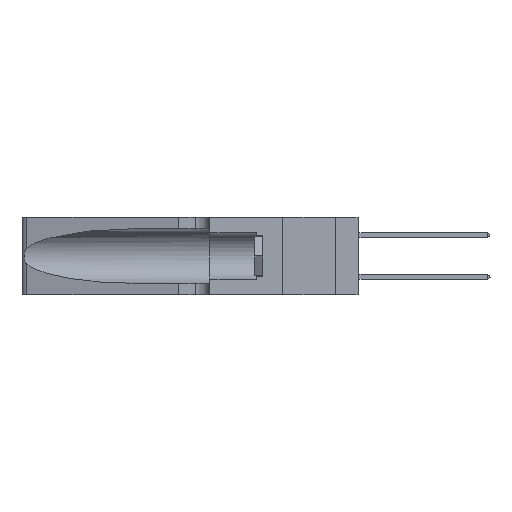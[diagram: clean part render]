
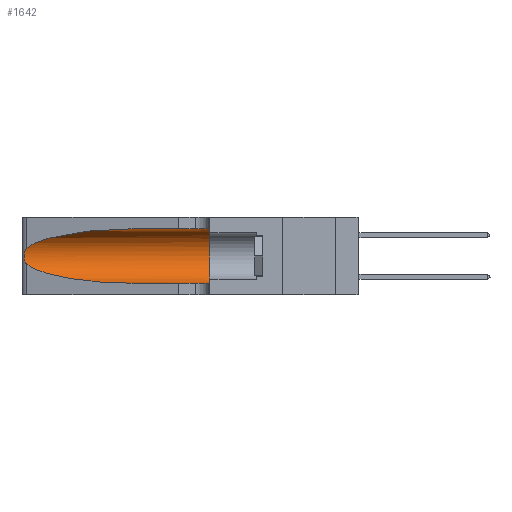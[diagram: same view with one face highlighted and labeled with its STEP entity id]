
A CAD part, left-side view. The second image highlights one B-rep face of the part: STEP entity #1642.
In plain terms, the highlighted cylindrical face has radius 3.308 mm (diameter 6.617 mm), a partial arc.
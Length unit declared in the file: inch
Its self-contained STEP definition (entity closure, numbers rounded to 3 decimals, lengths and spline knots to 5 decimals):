
#1467 = CARTESIAN_POINT ( 'NONE',  ( 0.25487, 1.22718, 0.14631 ) ) ;
#1642 = ADVANCED_FACE ( 'NONE', ( #1729 ), #6594, .F. ) ;
#1729 = FACE_OUTER_BOUND ( 'NONE', #39317, .T. ) ;
#2793 = CARTESIAN_POINT ( 'NONE',  ( 0.25856, 1.23593, 0.16098 ) ) ;
#3028 = EDGE_CURVE ( 'NONE', #35115, #24705, #32101, .T. ) ;
#3252 = CARTESIAN_POINT ( 'NONE',  ( 0.1305, 1.61858, 0.185 ) ) ;
#4493 = CARTESIAN_POINT ( 'NONE',  ( 0.25555, 1.22993, 0.14849 ) ) ;
#4665 = EDGE_CURVE ( 'NONE', #39613, #35115, #19788, .T. ) ;
#5432 = LINE ( 'NONE', #15049, #13195 ) ;
#6594 = CYLINDRICAL_SURFACE ( 'NONE', #13612, 0.13025 ) ;
#7009 =( BOUNDED_CURVE ( )  B_SPLINE_CURVE ( 3, ( #38324, #22607, #38751, #10418 ),
 .UNSPECIFIED., .F., .T. ) 
 B_SPLINE_CURVE_WITH_KNOTS ( ( 4, 4 ),
 ( 1.5708, 2.84003 ),
 .UNSPECIFIED. ) 
 CURVE ( )  GEOMETRIC_REPRESENTATION_ITEM ( )  RATIONAL_B_SPLINE_CURVE ( ( 1., 0.87, 0.87, 1. ) ) 
 REPRESENTATION_ITEM ( '' )  );
#7216 = CARTESIAN_POINT ( 'NONE',  ( 0.25487, 1.22718, 0.14631 ) ) ;
#8910 = LINE ( 'NONE', #9896, #18165 ) ;
#9599 = VERTEX_POINT ( 'NONE', #10794 ) ;
#9896 = CARTESIAN_POINT ( 'NONE',  ( 0.1305, 1.61858, 0.31525 ) ) ;
#10171 = DIRECTION ( 'NONE',  ( 0., -1., 0. ) ) ;
#10418 = CARTESIAN_POINT ( 'NONE',  ( 0.25487, 1.22718, 0.22369 ) ) ;
#10487 = CARTESIAN_POINT ( 'NONE',  ( 0.25639, 1.23186, 0.15144 ) ) ;
#10794 = CARTESIAN_POINT ( 'NONE',  ( 0.1305, 0.35, 0.05475 ) ) ;
#12109 = CARTESIAN_POINT ( 'NONE',  ( 0.25487, 1.22718, 0.14631 ) ) ;
#12225 = CARTESIAN_POINT ( 'NONE',  ( 0.1305, 0.35, 0.31525 ) ) ;
#12799 = DIRECTION ( 'NONE',  ( 0., 0., -1. ) ) ;
#12861 = EDGE_CURVE ( 'NONE', #25041, #39613, #7009, .T. ) ;
#12931 = EDGE_CURVE ( 'NONE', #17271, #9599, #18590, .T. ) ;
#13195 = VECTOR ( 'NONE', #28211, 39.37008 ) ;
#13612 = AXIS2_PLACEMENT_3D ( 'NONE', #3252, #37931, #12799 ) ;
#14173 = EDGE_CURVE ( 'NONE', #25041, #17271, #8910, .T. ) ;
#14566 = DIRECTION ( 'NONE',  ( 0., 0., 1. ) ) ;
#15049 = CARTESIAN_POINT ( 'NONE',  ( 0.1305, 1.61858, 0.05475 ) ) ;
#15365 = CARTESIAN_POINT ( 'NONE',  ( 0.18966, 0.96281, 0.05475 ) ) ;
#15463 = CARTESIAN_POINT ( 'NONE',  ( 0.26075, 1.23896, 0.178 ) ) ;
#15885 = EDGE_CURVE ( 'NONE', #24705, #9599, #5432, .T. ) ;
#16474 = AXIS2_PLACEMENT_3D ( 'NONE', #36719, #33332, #14566 ) ;
#17271 = VERTEX_POINT ( 'NONE', #12225 ) ;
#18165 = VECTOR ( 'NONE', #10171, 39.37008 ) ;
#18257 = ORIENTED_EDGE ( 'NONE', *, *, #12861, .T. ) ;
#18496 = CARTESIAN_POINT ( 'NONE',  ( 0.1305, 0.72297, 0.05475 ) ) ;
#18590 = CIRCLE ( 'NONE', #16474, 0.13025 ) ;
#19788 = B_SPLINE_CURVE_WITH_KNOTS ( 'NONE', 3,
 ( #38444, #26817, #24397, #38112, #36093, #34465, #34600, #15463, #37721, #2793, #30961, #10487, #4493, #7216 ),
 .UNSPECIFIED., .F., .F.,
 ( 4, 2, 2, 2, 2, 2, 4 ),
 ( 0., 0.00027, 0.00053, 0.00107, 0.0016, 0.00187, 0.00214 ),
 .UNSPECIFIED. ) ;
#21062 = ORIENTED_EDGE ( 'NONE', *, *, #15885, .T. ) ;
#22607 = CARTESIAN_POINT ( 'NONE',  ( 0.18966, 0.96281, 0.31525 ) ) ;
#24397 = CARTESIAN_POINT ( 'NONE',  ( 0.25639, 1.23184, 0.21858 ) ) ;
#24705 = VERTEX_POINT ( 'NONE', #36384 ) ;
#25041 = VERTEX_POINT ( 'NONE', #31755 ) ;
#26817 = CARTESIAN_POINT ( 'NONE',  ( 0.25555, 1.22994, 0.2215 ) ) ;
#27863 = CARTESIAN_POINT ( 'NONE',  ( 0.2373, 1.15595, 0.08982 ) ) ;
#28211 = DIRECTION ( 'NONE',  ( 0., -1., 0. ) ) ;
#30961 = CARTESIAN_POINT ( 'NONE',  ( 0.25789, 1.23486, 0.15765 ) ) ;
#31013 = ORIENTED_EDGE ( 'NONE', *, *, #12931, .F. ) ;
#31755 = CARTESIAN_POINT ( 'NONE',  ( 0.1305, 0.72297, 0.31525 ) ) ;
#32101 =( BOUNDED_CURVE ( )  B_SPLINE_CURVE ( 3, ( #12109, #27863, #15365, #18496 ),
 .UNSPECIFIED., .F., .T. ) 
 B_SPLINE_CURVE_WITH_KNOTS ( ( 4, 4 ),
 ( 3.44316, 4.71239 ),
 .UNSPECIFIED. ) 
 CURVE ( )  GEOMETRIC_REPRESENTATION_ITEM ( )  RATIONAL_B_SPLINE_CURVE ( ( 1., 0.87, 0.87, 1. ) ) 
 REPRESENTATION_ITEM ( '' )  );
#33243 = CARTESIAN_POINT ( 'NONE',  ( 0.25487, 1.22718, 0.22369 ) ) ;
#33322 = ORIENTED_EDGE ( 'NONE', *, *, #3028, .T. ) ;
#33332 = DIRECTION ( 'NONE',  ( 0., 1., 0. ) ) ;
#34465 = CARTESIAN_POINT ( 'NONE',  ( 0.26018, 1.23835, 0.19895 ) ) ;
#34600 = CARTESIAN_POINT ( 'NONE',  ( 0.26075, 1.23896, 0.19203 ) ) ;
#35115 = VERTEX_POINT ( 'NONE', #1467 ) ;
#36093 = CARTESIAN_POINT ( 'NONE',  ( 0.25854, 1.2359, 0.20912 ) ) ;
#36384 = CARTESIAN_POINT ( 'NONE',  ( 0.1305, 0.72297, 0.05475 ) ) ;
#36595 = ORIENTED_EDGE ( 'NONE', *, *, #14173, .F. ) ;
#36719 = CARTESIAN_POINT ( 'NONE',  ( 0.1305, 0.35, 0.185 ) ) ;
#37721 = CARTESIAN_POINT ( 'NONE',  ( 0.26017, 1.23833, 0.17102 ) ) ;
#37931 = DIRECTION ( 'NONE',  ( 0., -1., 0. ) ) ;
#38112 = CARTESIAN_POINT ( 'NONE',  ( 0.25787, 1.23484, 0.2124 ) ) ;
#38324 = CARTESIAN_POINT ( 'NONE',  ( 0.1305, 0.72297, 0.31525 ) ) ;
#38444 = CARTESIAN_POINT ( 'NONE',  ( 0.25487, 1.22718, 0.22369 ) ) ;
#38578 = ORIENTED_EDGE ( 'NONE', *, *, #4665, .T. ) ;
#38751 = CARTESIAN_POINT ( 'NONE',  ( 0.2373, 1.15595, 0.28018 ) ) ;
#39317 = EDGE_LOOP ( 'NONE', ( #18257, #38578, #33322, #21062, #31013, #36595 ) ) ;
#39613 = VERTEX_POINT ( 'NONE', #33243 ) ;
